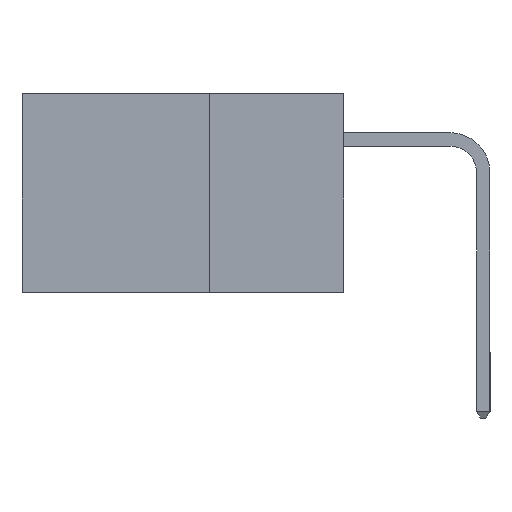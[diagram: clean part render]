
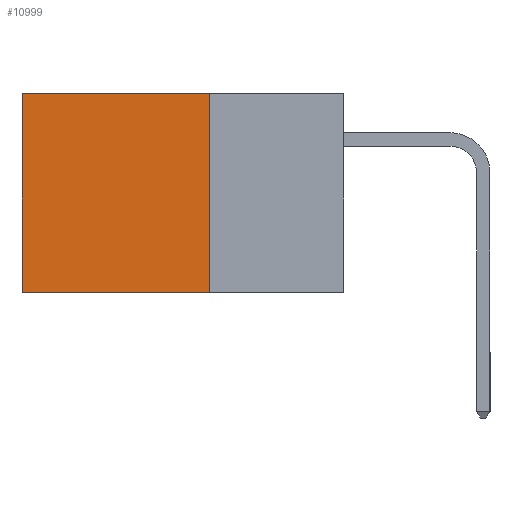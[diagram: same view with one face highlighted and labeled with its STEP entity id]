
A CAD part, left-side view. The second image highlights one B-rep face of the part: STEP entity #10999.
In plain terms, the highlighted planar face has unit normal (-1, 0, 0).
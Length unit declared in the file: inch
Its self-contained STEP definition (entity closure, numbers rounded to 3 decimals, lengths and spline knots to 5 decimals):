
#873 = DIRECTION ( 'NONE',  ( 0., 1., 0. ) ) ;
#1143 = DIRECTION ( 'NONE',  ( 0., 0., -1. ) ) ;
#1173 = ORIENTED_EDGE ( 'NONE', *, *, #11046, .T. ) ;
#1433 = DIRECTION ( 'NONE',  ( 0., 1., 0. ) ) ;
#1471 = CARTESIAN_POINT ( 'NONE',  ( 0.298, 0.6, 0. ) ) ;
#4380 = CARTESIAN_POINT ( 'NONE',  ( 0.298, 0.25, 0. ) ) ;
#4548 = ORIENTED_EDGE ( 'NONE', *, *, #14094, .F. ) ;
#5517 = LINE ( 'NONE', #7493, #6883 ) ;
#6069 = CARTESIAN_POINT ( 'NONE',  ( 0.298, 0.25, -0.37 ) ) ;
#6286 = LINE ( 'NONE', #20563, #22707 ) ;
#6883 = VECTOR ( 'NONE', #873, 39.37008 ) ;
#7370 = LINE ( 'NONE', #10302, #18593 ) ;
#7493 = CARTESIAN_POINT ( 'NONE',  ( 0.298, 0.25, 0. ) ) ;
#7603 = EDGE_CURVE ( 'NONE', #25170, #10013, #5517, .T. ) ;
#7720 = CARTESIAN_POINT ( 'NONE',  ( 0.298, 0.6, -0.37 ) ) ;
#8431 = LINE ( 'NONE', #10005, #16842 ) ;
#8823 = VERTEX_POINT ( 'NONE', #7720 ) ;
#9482 = DIRECTION ( 'NONE',  ( 0., 0., -1. ) ) ;
#9848 = FACE_OUTER_BOUND ( 'NONE', #28852, .T. ) ;
#9908 = DIRECTION ( 'NONE',  ( 1., 0., 0. ) ) ;
#10005 = CARTESIAN_POINT ( 'NONE',  ( 0.298, 0.6, 0. ) ) ;
#10013 = VERTEX_POINT ( 'NONE', #1471 ) ;
#10302 = CARTESIAN_POINT ( 'NONE',  ( 0.298, 0.25, -0.37 ) ) ;
#10999 = ADVANCED_FACE ( 'NONE', ( #9848 ), #14202, .F. ) ;
#11046 = EDGE_CURVE ( 'NONE', #10013, #8823, #8431, .T. ) ;
#13634 = EDGE_CURVE ( 'NONE', #23586, #8823, #7370, .T. ) ;
#14094 = EDGE_CURVE ( 'NONE', #25170, #23586, #6286, .T. ) ;
#14202 = PLANE ( 'NONE',  #20297 ) ;
#14302 = CARTESIAN_POINT ( 'NONE',  ( 0.298, 0.25, 0. ) ) ;
#16553 = ORIENTED_EDGE ( 'NONE', *, *, #7603, .T. ) ;
#16842 = VECTOR ( 'NONE', #1143, 39.37008 ) ;
#18593 = VECTOR ( 'NONE', #1433, 39.37008 ) ;
#19109 = DIRECTION ( 'NONE',  ( 0., 0., -1. ) ) ;
#20297 = AXIS2_PLACEMENT_3D ( 'NONE', #14302, #9908, #19109 ) ;
#20563 = CARTESIAN_POINT ( 'NONE',  ( 0.298, 0.25, 0. ) ) ;
#22324 = ORIENTED_EDGE ( 'NONE', *, *, #13634, .F. ) ;
#22707 = VECTOR ( 'NONE', #9482, 39.37008 ) ;
#23586 = VERTEX_POINT ( 'NONE', #6069 ) ;
#25170 = VERTEX_POINT ( 'NONE', #4380 ) ;
#28852 = EDGE_LOOP ( 'NONE', ( #1173, #22324, #4548, #16553 ) ) ;
